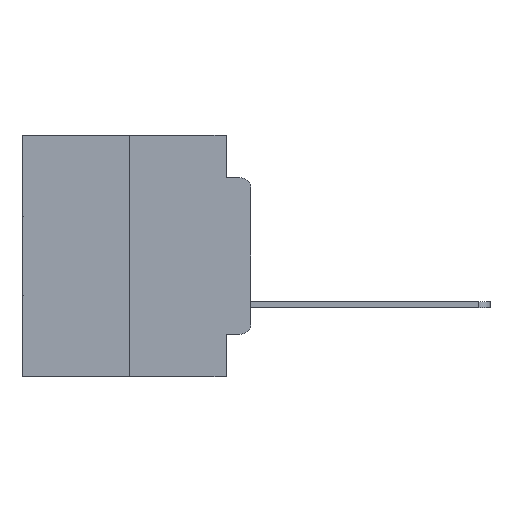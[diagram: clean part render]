
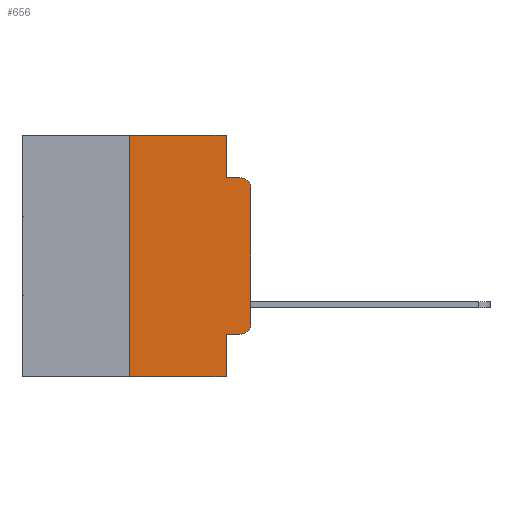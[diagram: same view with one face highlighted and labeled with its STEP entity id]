
A CAD part, left-side view. The second image highlights one B-rep face of the part: STEP entity #656.
In plain terms, the highlighted planar face has unit normal (-1, 0, 0).
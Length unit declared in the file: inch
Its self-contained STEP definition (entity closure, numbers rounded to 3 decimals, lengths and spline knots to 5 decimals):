
#450 = EDGE_CURVE ( 'NONE', #6488, #8596, #23580, .T. ) ;
#656 = ADVANCED_FACE ( 'NONE', ( #12558 ), #9952, .F. ) ;
#715 = LINE ( 'NONE', #26307, #17013 ) ;
#1033 = VERTEX_POINT ( 'NONE', #9954 ) ;
#1607 = LINE ( 'NONE', #30321, #4976 ) ;
#2165 = EDGE_CURVE ( 'NONE', #18816, #6488, #20095, .T. ) ;
#2242 = VERTEX_POINT ( 'NONE', #21333 ) ;
#2577 = ORIENTED_EDGE ( 'NONE', *, *, #19533, .T. ) ;
#2832 = EDGE_CURVE ( 'NONE', #2242, #18816, #10547, .T. ) ;
#3196 = VERTEX_POINT ( 'NONE', #23349 ) ;
#4113 = EDGE_CURVE ( 'NONE', #1033, #7442, #30770, .T. ) ;
#4493 = LINE ( 'NONE', #20250, #20775 ) ;
#4602 = DIRECTION ( 'NONE',  ( 0., 0., -1. ) ) ;
#4811 = CARTESIAN_POINT ( 'NONE',  ( 0., 0.051, -0.4115 ) ) ;
#4936 = ORIENTED_EDGE ( 'NONE', *, *, #2165, .F. ) ;
#4976 = VECTOR ( 'NONE', #10978, 39.37008 ) ;
#5018 = VECTOR ( 'NONE', #29177, 39.37008 ) ;
#6131 = DIRECTION ( 'NONE',  ( -1., 0., 0. ) ) ;
#6281 = ORIENTED_EDGE ( 'NONE', *, *, #14581, .F. ) ;
#6412 = CARTESIAN_POINT ( 'NONE',  ( 0., 0.051, -0.0885 ) ) ;
#6488 = VERTEX_POINT ( 'NONE', #6412 ) ;
#6493 = AXIS2_PLACEMENT_3D ( 'NONE', #22445, #24568, #26998 ) ;
#7442 = VERTEX_POINT ( 'NONE', #13042 ) ;
#7547 = CARTESIAN_POINT ( 'NONE',  ( 0., 0.051, 0. ) ) ;
#8151 = DIRECTION ( 'NONE',  ( 0., -1., 0. ) ) ;
#8596 = VERTEX_POINT ( 'NONE', #9904 ) ;
#8917 = CARTESIAN_POINT ( 'NONE',  ( 0., 0.051, -0.0885 ) ) ;
#9904 = CARTESIAN_POINT ( 'NONE',  ( 0., 0.02, -0.0885 ) ) ;
#9952 = PLANE ( 'NONE',  #6493 ) ;
#9954 = CARTESIAN_POINT ( 'NONE',  ( 0., 0., -0.3915 ) ) ;
#10048 = ORIENTED_EDGE ( 'NONE', *, *, #2832, .F. ) ;
#10547 = LINE ( 'NONE', #14092, #29105 ) ;
#10978 = DIRECTION ( 'NONE',  ( 0., 0., 1. ) ) ;
#11664 = DIRECTION ( 'NONE',  ( 0., -1., 0. ) ) ;
#12345 = CARTESIAN_POINT ( 'NONE',  ( 0., 0.02, -0.3915 ) ) ;
#12558 = FACE_OUTER_BOUND ( 'NONE', #15307, .T. ) ;
#12946 = DIRECTION ( 'NONE',  ( 0., -1., 0. ) ) ;
#13042 = CARTESIAN_POINT ( 'NONE',  ( 0., 0., -0.1085 ) ) ;
#13628 = VECTOR ( 'NONE', #14028, 39.37008 ) ;
#13771 = VERTEX_POINT ( 'NONE', #14322 ) ;
#14028 = DIRECTION ( 'NONE',  ( 0., 0., -1. ) ) ;
#14092 = CARTESIAN_POINT ( 'NONE',  ( 0., 0.473, 0. ) ) ;
#14322 = CARTESIAN_POINT ( 'NONE',  ( 0., 0.051, -0.5 ) ) ;
#14581 = EDGE_CURVE ( 'NONE', #28420, #2242, #1607, .T. ) ;
#15307 = EDGE_LOOP ( 'NONE', ( #24445, #2577, #23798, #4936, #10048, #6281, #25504, #26190, #16090, #27509 ) ) ;
#16090 = ORIENTED_EDGE ( 'NONE', *, *, #29359, .T. ) ;
#17013 = VECTOR ( 'NONE', #4602, 39.37008 ) ;
#17954 = AXIS2_PLACEMENT_3D ( 'NONE', #12345, #21778, #19435 ) ;
#18816 = VERTEX_POINT ( 'NONE', #7547 ) ;
#19435 = DIRECTION ( 'NONE',  ( 0., 0., -1. ) ) ;
#19453 = CARTESIAN_POINT ( 'NONE',  ( 0., 0., 0. ) ) ;
#19533 = EDGE_CURVE ( 'NONE', #7442, #8596, #25670, .T. ) ;
#20095 = LINE ( 'NONE', #30921, #13628 ) ;
#20250 = CARTESIAN_POINT ( 'NONE',  ( 0., 0.051, -0.4115 ) ) ;
#20775 = VECTOR ( 'NONE', #8151, 39.37008 ) ;
#21333 = CARTESIAN_POINT ( 'NONE',  ( 0., 0.25, 0. ) ) ;
#21778 = DIRECTION ( 'NONE',  ( -1., 0., 0. ) ) ;
#22181 = AXIS2_PLACEMENT_3D ( 'NONE', #23199, #6131, #27735 ) ;
#22445 = CARTESIAN_POINT ( 'NONE',  ( 0., 0.473, 0. ) ) ;
#22782 = CARTESIAN_POINT ( 'NONE',  ( 0., 0.473, -0.5 ) ) ;
#23199 = CARTESIAN_POINT ( 'NONE',  ( 0., 0.02, -0.1085 ) ) ;
#23349 = CARTESIAN_POINT ( 'NONE',  ( 0., 0.02, -0.4115 ) ) ;
#23580 = LINE ( 'NONE', #8917, #24697 ) ;
#23798 = ORIENTED_EDGE ( 'NONE', *, *, #450, .F. ) ;
#24445 = ORIENTED_EDGE ( 'NONE', *, *, #4113, .T. ) ;
#24568 = DIRECTION ( 'NONE',  ( 1., 0., 0. ) ) ;
#24697 = VECTOR ( 'NONE', #30279, 39.37008 ) ;
#25504 = ORIENTED_EDGE ( 'NONE', *, *, #25532, .T. ) ;
#25532 = EDGE_CURVE ( 'NONE', #28420, #13771, #27968, .T. ) ;
#25670 = CIRCLE ( 'NONE', #22181, 0.02 ) ;
#26190 = ORIENTED_EDGE ( 'NONE', *, *, #29136, .F. ) ;
#26307 = CARTESIAN_POINT ( 'NONE',  ( 0., 0.051, 0. ) ) ;
#26339 = CARTESIAN_POINT ( 'NONE',  ( 0., 0.25, -0.5 ) ) ;
#26460 = VECTOR ( 'NONE', #12946, 39.37008 ) ;
#26998 = DIRECTION ( 'NONE',  ( 0., 0., -1. ) ) ;
#27509 = ORIENTED_EDGE ( 'NONE', *, *, #30420, .T. ) ;
#27735 = DIRECTION ( 'NONE',  ( 0., 0., -1. ) ) ;
#27968 = LINE ( 'NONE', #22782, #26460 ) ;
#28420 = VERTEX_POINT ( 'NONE', #26339 ) ;
#29016 = CIRCLE ( 'NONE', #17954, 0.02 ) ;
#29105 = VECTOR ( 'NONE', #11664, 39.37008 ) ;
#29136 = EDGE_CURVE ( 'NONE', #30406, #13771, #715, .T. ) ;
#29177 = DIRECTION ( 'NONE',  ( 0., 0., 1. ) ) ;
#29359 = EDGE_CURVE ( 'NONE', #30406, #3196, #4493, .T. ) ;
#30279 = DIRECTION ( 'NONE',  ( 0., -1., 0. ) ) ;
#30321 = CARTESIAN_POINT ( 'NONE',  ( 0., 0.25, 0. ) ) ;
#30406 = VERTEX_POINT ( 'NONE', #4811 ) ;
#30420 = EDGE_CURVE ( 'NONE', #3196, #1033, #29016, .T. ) ;
#30770 = LINE ( 'NONE', #19453, #5018 ) ;
#30921 = CARTESIAN_POINT ( 'NONE',  ( 0., 0.051, 0. ) ) ;
